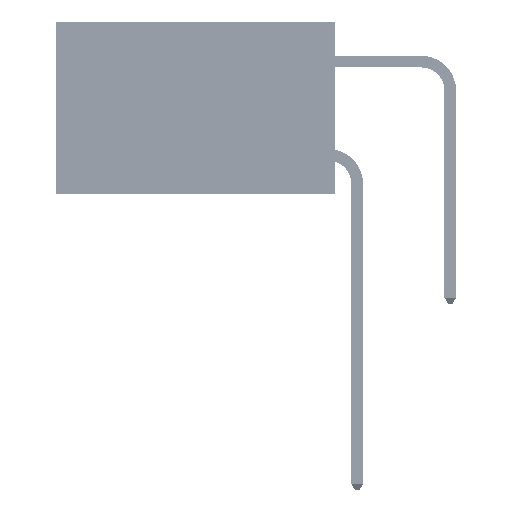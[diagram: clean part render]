
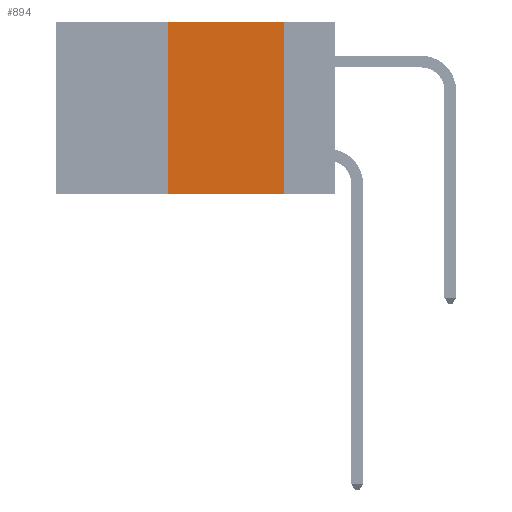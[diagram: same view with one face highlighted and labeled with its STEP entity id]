
A CAD part, left-side view. The second image highlights one B-rep face of the part: STEP entity #894.
In plain terms, the highlighted planar face has unit normal (-1, 0, 0).
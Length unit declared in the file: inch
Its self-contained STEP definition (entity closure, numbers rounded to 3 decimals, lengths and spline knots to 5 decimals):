
#894 = ADVANCED_FACE ( 'NONE', ( #2009 ), #3505, .F. ) ;
#1516 = AXIS2_PLACEMENT_3D ( 'NONE', #23455, #47184, #7591 ) ;
#1573 = CARTESIAN_POINT ( 'NONE',  ( 0., 0.36, 0. ) ) ;
#2009 = FACE_OUTER_BOUND ( 'NONE', #15945, .T. ) ;
#2338 = ORIENTED_EDGE ( 'NONE', *, *, #14513, .F. ) ;
#2583 = CARTESIAN_POINT ( 'NONE',  ( 0., 0.6, 0. ) ) ;
#2902 = CARTESIAN_POINT ( 'NONE',  ( 0., 0.11, 0. ) ) ;
#3505 = PLANE ( 'NONE',  #1516 ) ;
#6901 = VECTOR ( 'NONE', #9758, 39.37008 ) ;
#7591 = DIRECTION ( 'NONE',  ( 0., 0., -1. ) ) ;
#7746 = CARTESIAN_POINT ( 'NONE',  ( 0., 0.11, 0. ) ) ;
#9758 = DIRECTION ( 'NONE',  ( 0., 0., 1. ) ) ;
#12415 = CARTESIAN_POINT ( 'NONE',  ( 0., 0.36, 0. ) ) ;
#13630 = VECTOR ( 'NONE', #51423, 39.37008 ) ;
#14513 = EDGE_CURVE ( 'NONE', #47523, #40430, #15447, .T. ) ;
#15447 = LINE ( 'NONE', #2583, #16721 ) ;
#15945 = EDGE_LOOP ( 'NONE', ( #22442, #2338, #34275, #47212 ) ) ;
#15963 = EDGE_CURVE ( 'NONE', #19844, #47523, #17597, .T. ) ;
#16721 = VECTOR ( 'NONE', #30553, 39.37008 ) ;
#16732 = DIRECTION ( 'NONE',  ( 0., -1., 0. ) ) ;
#17597 = LINE ( 'NONE', #1573, #6901 ) ;
#18779 = CARTESIAN_POINT ( 'NONE',  ( 0., 0.36, -0.37 ) ) ;
#19844 = VERTEX_POINT ( 'NONE', #18779 ) ;
#20789 = CARTESIAN_POINT ( 'NONE',  ( 0., 0.11, -0.37 ) ) ;
#22442 = ORIENTED_EDGE ( 'NONE', *, *, #31922, .F. ) ;
#23455 = CARTESIAN_POINT ( 'NONE',  ( 0., 0.6, 0. ) ) ;
#24158 = LINE ( 'NONE', #7746, #13630 ) ;
#24816 = LINE ( 'NONE', #36544, #34201 ) ;
#30553 = DIRECTION ( 'NONE',  ( 0., -1., 0. ) ) ;
#31922 = EDGE_CURVE ( 'NONE', #40430, #50508, #24158, .T. ) ;
#34201 = VECTOR ( 'NONE', #16732, 39.37008 ) ;
#34275 = ORIENTED_EDGE ( 'NONE', *, *, #15963, .F. ) ;
#36544 = CARTESIAN_POINT ( 'NONE',  ( 0., 0.6, -0.37 ) ) ;
#40430 = VERTEX_POINT ( 'NONE', #2902 ) ;
#46184 = EDGE_CURVE ( 'NONE', #19844, #50508, #24816, .T. ) ;
#47184 = DIRECTION ( 'NONE',  ( 1., 0., 0. ) ) ;
#47212 = ORIENTED_EDGE ( 'NONE', *, *, #46184, .T. ) ;
#47523 = VERTEX_POINT ( 'NONE', #12415 ) ;
#50508 = VERTEX_POINT ( 'NONE', #20789 ) ;
#51423 = DIRECTION ( 'NONE',  ( 0., 0., -1. ) ) ;
